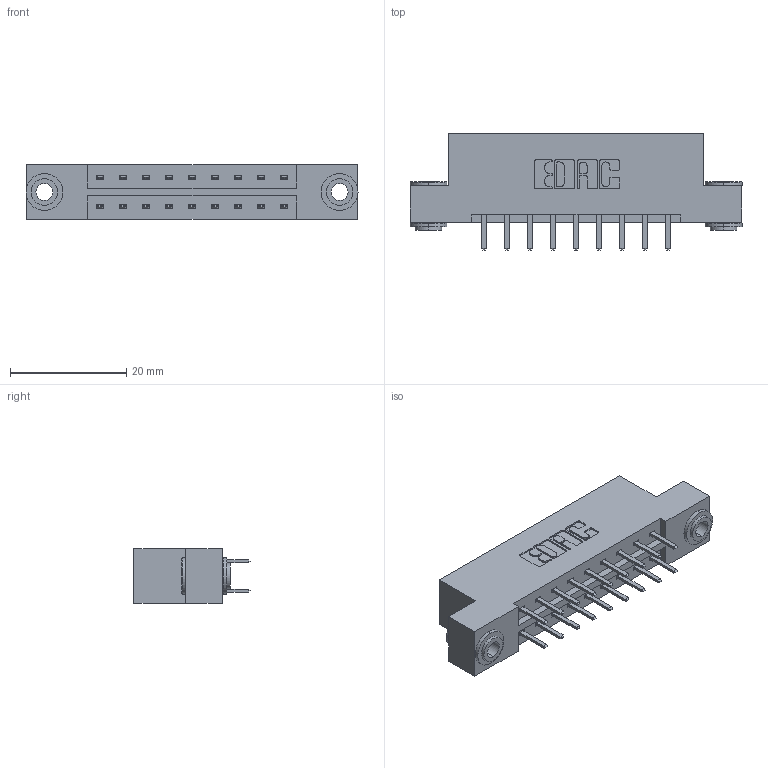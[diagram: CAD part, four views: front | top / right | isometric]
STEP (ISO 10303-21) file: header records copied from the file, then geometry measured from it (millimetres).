
FILE_DESCRIPTION (( 'STEP AP203' ), '1' );
FILE_NAME ('833-018-520-203.STEP', '2020-05-31T21:02:10', ( '' ), ( '' ), 'SwSTEP 2.0', 'SolidWorks 2020', '' );
FILE_SCHEMA (( 'CONFIG_CONTROL_DESIGN' ));
Length unit declared in the file: inch
Products named in the file (4): 833 Part_Flush - .156 Dia - TH; 345-250-002_345-250-002-102; 345-292-001_345-293-120; 833-018-520-203
Assembly tree (21 placements, depth 2):
  833-018-520-203
    833 Part_Flush - .156 Dia - TH
    345-292-001_345-293-120  x18
    345-250-002_345-250-002-102  x2
Bounding box: 57.2 x 20.02 x 9.4 mm (x, y, z)
Volume: 5542.7 mm3; surface area: 6398.2 mm2
Topology: 21 solids, 21 shells, 1160 faces, 3321 edges, 2162 vertices
Faces by surface type: plane 764, cylinder 388, cone 8
Entity records: 10822 total; most frequent: CARTESIAN_POINT 1821, ORIENTED_EDGE 1738, DIRECTION 1635, EDGE_CURVE 869, LINE 713, VECTOR 713, VERTEX_POINT 574, AXIS2_PLACEMENT_3D 461
